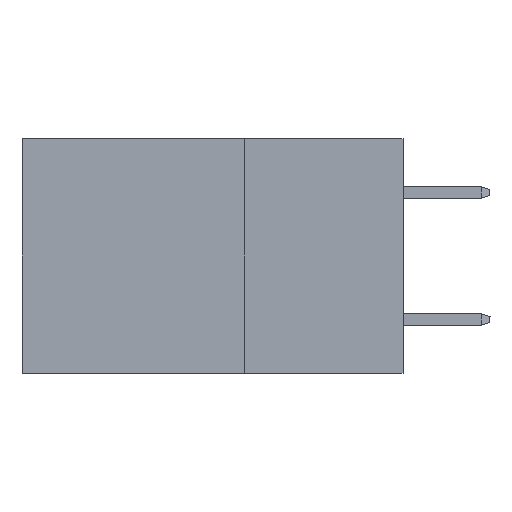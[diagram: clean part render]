
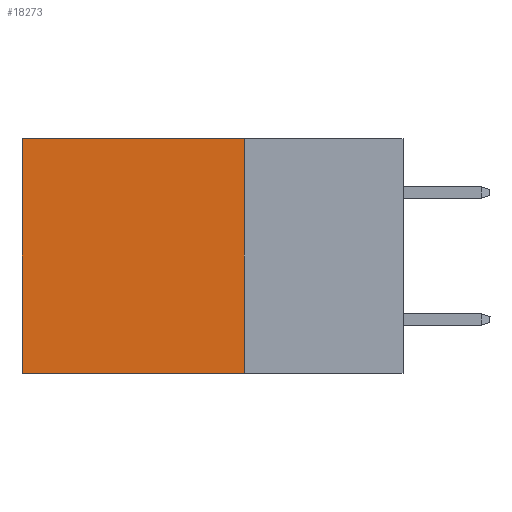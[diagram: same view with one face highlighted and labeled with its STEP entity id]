
A CAD part, left-side view. The second image highlights one B-rep face of the part: STEP entity #18273.
In plain terms, the highlighted planar face has unit normal (-1, 0, 0).
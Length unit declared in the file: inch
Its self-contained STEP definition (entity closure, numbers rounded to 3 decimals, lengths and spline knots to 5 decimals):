
#2767 = VECTOR ( 'NONE', #30219, 39.37008 ) ;
#3265 = EDGE_CURVE ( 'NONE', #28253, #22663, #8594, .T. ) ;
#3404 = VERTEX_POINT ( 'NONE', #21102 ) ;
#5597 = EDGE_CURVE ( 'NONE', #28253, #26683, #6362, .T. ) ;
#5943 = EDGE_LOOP ( 'NONE', ( #20604, #7262, #30166, #21156 ) ) ;
#6296 = DIRECTION ( 'NONE',  ( 1., 0., 0. ) ) ;
#6362 = LINE ( 'NONE', #15922, #25948 ) ;
#7262 = ORIENTED_EDGE ( 'NONE', *, *, #23359, .F. ) ;
#8440 = CARTESIAN_POINT ( 'NONE',  ( 0.2875, 0.25, 0. ) ) ;
#8594 = LINE ( 'NONE', #8440, #2767 ) ;
#9337 = DIRECTION ( 'NONE',  ( 0., 0., -1. ) ) ;
#13826 = CARTESIAN_POINT ( 'NONE',  ( 0.2875, 0.25, -0.37 ) ) ;
#13888 = VECTOR ( 'NONE', #15737, 39.37008 ) ;
#14333 = CARTESIAN_POINT ( 'NONE',  ( 0.2875, 0.25, 0. ) ) ;
#15574 = LINE ( 'NONE', #30021, #13888 ) ;
#15737 = DIRECTION ( 'NONE',  ( 0., 1., 0. ) ) ;
#15922 = CARTESIAN_POINT ( 'NONE',  ( 0.2875, 0.25, 0. ) ) ;
#18195 = FACE_OUTER_BOUND ( 'NONE', #5943, .T. ) ;
#18273 = ADVANCED_FACE ( 'NONE', ( #18195 ), #24781, .F. ) ;
#20604 = ORIENTED_EDGE ( 'NONE', *, *, #20659, .T. ) ;
#20659 = EDGE_CURVE ( 'NONE', #26683, #3404, #25651, .T. ) ;
#21102 = CARTESIAN_POINT ( 'NONE',  ( 0.2875, 0.6, -0.37 ) ) ;
#21156 = ORIENTED_EDGE ( 'NONE', *, *, #5597, .T. ) ;
#22524 = CARTESIAN_POINT ( 'NONE',  ( 0.2875, 0.6, 0. ) ) ;
#22663 = VERTEX_POINT ( 'NONE', #13826 ) ;
#23359 = EDGE_CURVE ( 'NONE', #22663, #3404, #15574, .T. ) ;
#24781 = PLANE ( 'NONE',  #30731 ) ;
#25416 = DIRECTION ( 'NONE',  ( 0., 0., -1. ) ) ;
#25651 = LINE ( 'NONE', #26114, #25745 ) ;
#25745 = VECTOR ( 'NONE', #9337, 39.37008 ) ;
#25948 = VECTOR ( 'NONE', #28006, 39.37008 ) ;
#26114 = CARTESIAN_POINT ( 'NONE',  ( 0.2875, 0.6, 0. ) ) ;
#26683 = VERTEX_POINT ( 'NONE', #22524 ) ;
#27797 = CARTESIAN_POINT ( 'NONE',  ( 0.2875, 0.25, 0. ) ) ;
#28006 = DIRECTION ( 'NONE',  ( 0., 1., 0. ) ) ;
#28253 = VERTEX_POINT ( 'NONE', #14333 ) ;
#30021 = CARTESIAN_POINT ( 'NONE',  ( 0.2875, 0.25, -0.37 ) ) ;
#30166 = ORIENTED_EDGE ( 'NONE', *, *, #3265, .F. ) ;
#30219 = DIRECTION ( 'NONE',  ( 0., 0., -1. ) ) ;
#30731 = AXIS2_PLACEMENT_3D ( 'NONE', #27797, #6296, #25416 ) ;
